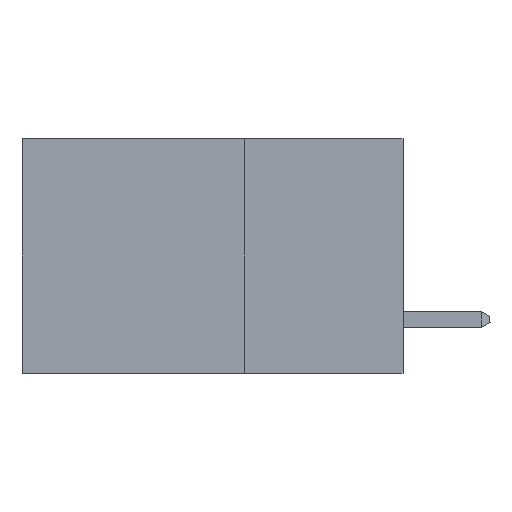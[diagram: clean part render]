
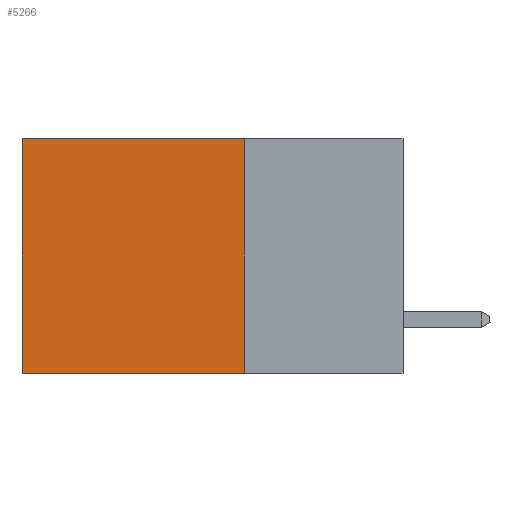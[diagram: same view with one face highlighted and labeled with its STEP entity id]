
A CAD part, left-side view. The second image highlights one B-rep face of the part: STEP entity #5266.
In plain terms, the highlighted planar face has unit normal (-1, 0, 0).
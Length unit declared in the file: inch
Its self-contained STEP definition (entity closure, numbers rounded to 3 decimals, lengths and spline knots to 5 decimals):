
#428 = ORIENTED_EDGE ( 'NONE', *, *, #3768, .T. ) ;
#795 = CARTESIAN_POINT ( 'NONE',  ( 0.2875, 0.25, -0.37 ) ) ;
#1617 = CARTESIAN_POINT ( 'NONE',  ( 0.2875, 0.25, 0. ) ) ;
#2870 = DIRECTION ( 'NONE',  ( 0., 1., 0. ) ) ;
#3075 = VERTEX_POINT ( 'NONE', #25035 ) ;
#3768 = EDGE_CURVE ( 'NONE', #5927, #17079, #6635, .T. ) ;
#4566 = CARTESIAN_POINT ( 'NONE',  ( 0.2875, 0.6, 0. ) ) ;
#5208 = VECTOR ( 'NONE', #10195, 39.37008 ) ;
#5266 = ADVANCED_FACE ( 'NONE', ( #13504 ), #6536, .F. ) ;
#5927 = VERTEX_POINT ( 'NONE', #11043 ) ;
#6305 = VECTOR ( 'NONE', #16746, 39.37008 ) ;
#6416 = CARTESIAN_POINT ( 'NONE',  ( 0.2875, 0.25, 0. ) ) ;
#6536 = PLANE ( 'NONE',  #22514 ) ;
#6635 = LINE ( 'NONE', #6416, #6305 ) ;
#6820 = DIRECTION ( 'NONE',  ( 0., 0., -1. ) ) ;
#8942 = CARTESIAN_POINT ( 'NONE',  ( 0.2875, 0.25, 0. ) ) ;
#9032 = CARTESIAN_POINT ( 'NONE',  ( 0.2875, 0.25, -0.37 ) ) ;
#9800 = ORIENTED_EDGE ( 'NONE', *, *, #16286, .F. ) ;
#10195 = DIRECTION ( 'NONE',  ( 0., 0., -1. ) ) ;
#10835 = VECTOR ( 'NONE', #2870, 39.37008 ) ;
#11043 = CARTESIAN_POINT ( 'NONE',  ( 0.2875, 0.25, 0. ) ) ;
#11214 = LINE ( 'NONE', #795, #10835 ) ;
#13053 = CARTESIAN_POINT ( 'NONE',  ( 0.2875, 0.6, 0. ) ) ;
#13504 = FACE_OUTER_BOUND ( 'NONE', #23114, .T. ) ;
#14071 = LINE ( 'NONE', #13053, #19278 ) ;
#15135 = DIRECTION ( 'NONE',  ( 1., 0., 0. ) ) ;
#16286 = EDGE_CURVE ( 'NONE', #5927, #20142, #16425, .T. ) ;
#16425 = LINE ( 'NONE', #1617, #5208 ) ;
#16746 = DIRECTION ( 'NONE',  ( 0., 1., 0. ) ) ;
#17079 = VERTEX_POINT ( 'NONE', #4566 ) ;
#18452 = EDGE_CURVE ( 'NONE', #17079, #3075, #14071, .T. ) ;
#19278 = VECTOR ( 'NONE', #19575, 39.37008 ) ;
#19575 = DIRECTION ( 'NONE',  ( 0., 0., -1. ) ) ;
#20142 = VERTEX_POINT ( 'NONE', #9032 ) ;
#21927 = ORIENTED_EDGE ( 'NONE', *, *, #24805, .F. ) ;
#22363 = ORIENTED_EDGE ( 'NONE', *, *, #18452, .T. ) ;
#22514 = AXIS2_PLACEMENT_3D ( 'NONE', #8942, #15135, #6820 ) ;
#23114 = EDGE_LOOP ( 'NONE', ( #22363, #21927, #9800, #428 ) ) ;
#24805 = EDGE_CURVE ( 'NONE', #20142, #3075, #11214, .T. ) ;
#25035 = CARTESIAN_POINT ( 'NONE',  ( 0.2875, 0.6, -0.37 ) ) ;
